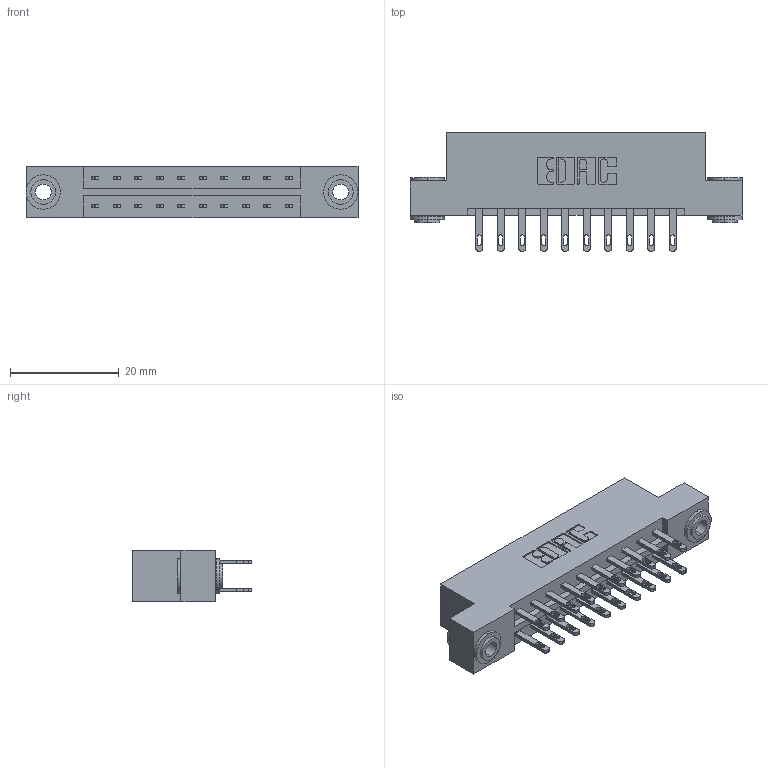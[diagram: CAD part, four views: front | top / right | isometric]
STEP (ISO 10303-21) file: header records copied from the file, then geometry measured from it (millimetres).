
FILE_DESCRIPTION (( 'STEP AP203' ), '1' );
FILE_NAME ('833-020-500-203.STEP', '2020-06-01T01:13:33', ( '' ), ( '' ), 'SwSTEP 2.0', 'SolidWorks 2020', '' );
FILE_SCHEMA (( 'CONFIG_CONTROL_DESIGN' ));
Length unit declared in the file: inch
Products named in the file (4): 345-292-001_345-293-100; 833-020-500-203; 345-250-002_345-250-002-102; 833 Part_Flush - .156 Dia - TH
Assembly tree (23 placements, depth 2):
  833-020-500-203
    833 Part_Flush - .156 Dia - TH
    345-292-001_345-293-100  x20
    345-250-002_345-250-002-102  x2
Bounding box: 61.16 x 21.85 x 9.4 mm (x, y, z)
Volume: 6025.7 mm3; surface area: 7221 mm2
Topology: 23 solids, 23 shells, 1112 faces, 3327 edges, 2214 vertices
Faces by surface type: plane 680, cylinder 424, cone 8
Entity records: 11152 total; most frequent: CARTESIAN_POINT 1861, ORIENTED_EDGE 1790, DIRECTION 1681, EDGE_CURVE 895, VECTOR 739, LINE 739, VERTEX_POINT 594, AXIS2_PLACEMENT_3D 471
